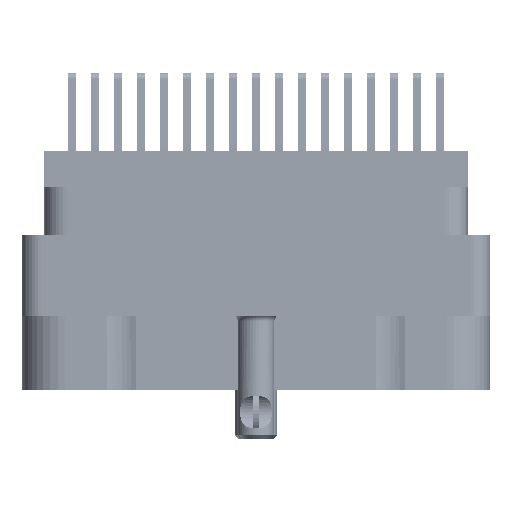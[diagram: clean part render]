
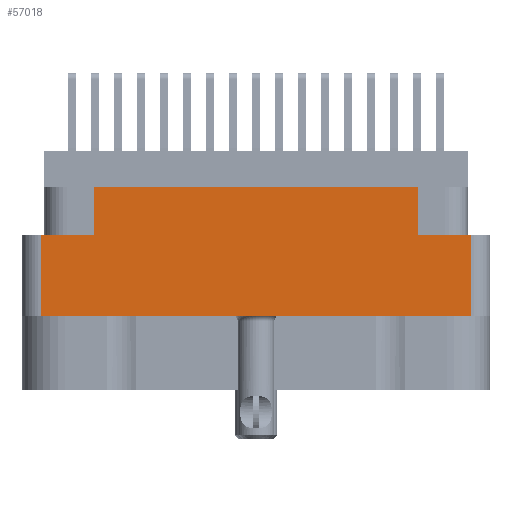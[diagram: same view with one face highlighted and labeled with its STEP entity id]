
A CAD part, left-side view. The second image highlights one B-rep face of the part: STEP entity #57018.
In plain terms, the highlighted planar face has unit normal (-1, 0, 0).
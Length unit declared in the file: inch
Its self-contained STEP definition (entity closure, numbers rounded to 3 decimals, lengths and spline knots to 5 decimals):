
#1732 = VECTOR ( 'NONE', #34322, 39.37008 ) ;
#6459 = EDGE_CURVE ( 'NONE', #21034, #74538, #68739, .T. ) ;
#8320 = CARTESIAN_POINT ( 'NONE',  ( -1.375, 0.7005, -0.274 ) ) ;
#10397 = CARTESIAN_POINT ( 'NONE',  ( -1.375, 0., -0.274 ) ) ;
#13356 = ORIENTED_EDGE ( 'NONE', *, *, #21244, .F. ) ;
#13843 = VERTEX_POINT ( 'NONE', #92460 ) ;
#15541 = EDGE_CURVE ( 'NONE', #45708, #78290, #20785, .T. ) ;
#16025 = ORIENTED_EDGE ( 'NONE', *, *, #6459, .F. ) ;
#16185 = CARTESIAN_POINT ( 'NONE',  ( -1.375, -0.7005, -0.54 ) ) ;
#16937 = ORIENTED_EDGE ( 'NONE', *, *, #57902, .T. ) ;
#17285 = LINE ( 'NONE', #98978, #35513 ) ;
#17383 = CARTESIAN_POINT ( 'NONE',  ( -1.375, 0.7005, -0.78 ) ) ;
#17749 = CARTESIAN_POINT ( 'NONE',  ( -1.375, -0.7005, -0.78 ) ) ;
#20580 = ORIENTED_EDGE ( 'NONE', *, *, #24032, .T. ) ;
#20785 = LINE ( 'NONE', #17749, #54813 ) ;
#21034 = VERTEX_POINT ( 'NONE', #52047 ) ;
#21244 = EDGE_CURVE ( 'NONE', #67773, #78290, #69608, .T. ) ;
#22397 = LINE ( 'NONE', #50206, #33278 ) ;
#23581 = VECTOR ( 'NONE', #83752, 39.37008 ) ;
#24032 = EDGE_CURVE ( 'NONE', #52870, #13843, #75733, .T. ) ;
#24069 = CARTESIAN_POINT ( 'NONE',  ( -1.375, -0.5285, -0.274 ) ) ;
#26560 = CARTESIAN_POINT ( 'NONE',  ( -1.375, 0., -0.54 ) ) ;
#26568 = DIRECTION ( 'NONE',  ( 0., 0., -1. ) ) ;
#26756 = VERTEX_POINT ( 'NONE', #72147 ) ;
#31744 = AXIS2_PLACEMENT_3D ( 'NONE', #75568, #50808, #98665 ) ;
#33278 = VECTOR ( 'NONE', #42354, 39.37008 ) ;
#33301 = LINE ( 'NONE', #92249, #23581 ) ;
#34322 = DIRECTION ( 'NONE',  ( 0., -1., 0. ) ) ;
#35513 = VECTOR ( 'NONE', #52444, 39.37008 ) ;
#37406 = CARTESIAN_POINT ( 'NONE',  ( -1.375, 0.7625, -0.117 ) ) ;
#37857 = CARTESIAN_POINT ( 'NONE',  ( -1.375, -0.5285, -0.117 ) ) ;
#38605 = ORIENTED_EDGE ( 'NONE', *, *, #15541, .T. ) ;
#40878 = CARTESIAN_POINT ( 'NONE',  ( -1.375, -0.7005, -0.274 ) ) ;
#42354 = DIRECTION ( 'NONE',  ( 0., 0., 1. ) ) ;
#45708 = VERTEX_POINT ( 'NONE', #16185 ) ;
#46123 = EDGE_CURVE ( 'NONE', #67773, #74538, #33301, .T. ) ;
#46587 = VECTOR ( 'NONE', #26568, 39.37008 ) ;
#50206 = CARTESIAN_POINT ( 'NONE',  ( -1.375, 0.5285, -0.274 ) ) ;
#50808 = DIRECTION ( 'NONE',  ( -1., 0., 0. ) ) ;
#52047 = CARTESIAN_POINT ( 'NONE',  ( -1.375, 0.5285, -0.117 ) ) ;
#52444 = DIRECTION ( 'NONE',  ( 0., -1., 0. ) ) ;
#52870 = VERTEX_POINT ( 'NONE', #8320 ) ;
#54813 = VECTOR ( 'NONE', #79919, 39.37008 ) ;
#56781 = EDGE_CURVE ( 'NONE', #26756, #21034, #22397, .T. ) ;
#57018 = ADVANCED_FACE ( 'NONE', ( #66006 ), #98008, .T. ) ;
#57705 = DIRECTION ( 'NONE',  ( 0., -1., 0. ) ) ;
#57902 = EDGE_CURVE ( 'NONE', #13843, #45708, #70983, .T. ) ;
#60856 = DIRECTION ( 'NONE',  ( 0., -1., 0. ) ) ;
#66006 = FACE_OUTER_BOUND ( 'NONE', #78264, .T. ) ;
#67185 = VECTOR ( 'NONE', #57705, 39.37008 ) ;
#67773 = VERTEX_POINT ( 'NONE', #24069 ) ;
#68739 = LINE ( 'NONE', #37406, #73659 ) ;
#69608 = LINE ( 'NONE', #10397, #67185 ) ;
#70983 = LINE ( 'NONE', #26560, #1732 ) ;
#72147 = CARTESIAN_POINT ( 'NONE',  ( -1.375, 0.5285, -0.274 ) ) ;
#73659 = VECTOR ( 'NONE', #60856, 39.37008 ) ;
#74538 = VERTEX_POINT ( 'NONE', #37857 ) ;
#75568 = CARTESIAN_POINT ( 'NONE',  ( -1.375, -0.7625, -0.78 ) ) ;
#75733 = LINE ( 'NONE', #17383, #46587 ) ;
#76369 = ORIENTED_EDGE ( 'NONE', *, *, #56781, .F. ) ;
#78264 = EDGE_LOOP ( 'NONE', ( #100681, #20580, #16937, #38605, #13356, #83382, #16025, #76369 ) ) ;
#78290 = VERTEX_POINT ( 'NONE', #40878 ) ;
#78492 = EDGE_CURVE ( 'NONE', #52870, #26756, #17285, .T. ) ;
#79919 = DIRECTION ( 'NONE',  ( 0., 0., 1. ) ) ;
#83382 = ORIENTED_EDGE ( 'NONE', *, *, #46123, .T. ) ;
#83752 = DIRECTION ( 'NONE',  ( 0., 0., 1. ) ) ;
#92249 = CARTESIAN_POINT ( 'NONE',  ( -1.375, -0.5285, -0.274 ) ) ;
#92460 = CARTESIAN_POINT ( 'NONE',  ( -1.375, 0.7005, -0.54 ) ) ;
#98008 = PLANE ( 'NONE',  #31744 ) ;
#98665 = DIRECTION ( 'NONE',  ( 0., 0., 1. ) ) ;
#98978 = CARTESIAN_POINT ( 'NONE',  ( -1.375, 0., -0.274 ) ) ;
#100681 = ORIENTED_EDGE ( 'NONE', *, *, #78492, .F. ) ;
